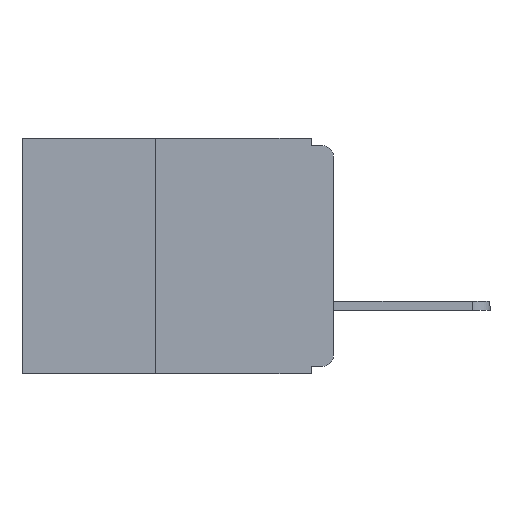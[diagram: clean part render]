
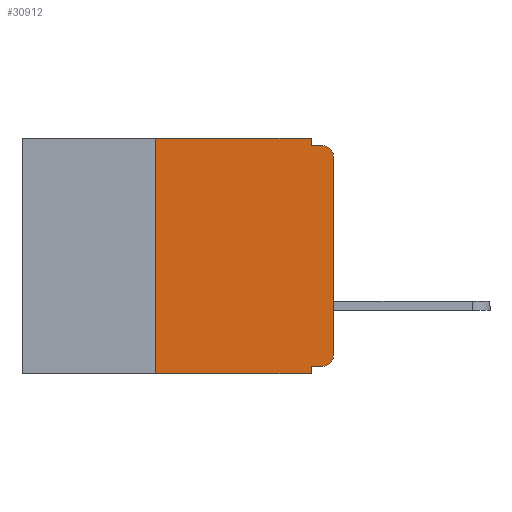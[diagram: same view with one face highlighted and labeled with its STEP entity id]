
A CAD part, left-side view. The second image highlights one B-rep face of the part: STEP entity #30912.
In plain terms, the highlighted planar face has unit normal (-1, 0, 0).
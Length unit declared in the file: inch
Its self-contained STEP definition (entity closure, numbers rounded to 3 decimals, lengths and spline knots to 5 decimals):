
#109 = VECTOR ( 'NONE', #897, 39.37008 ) ;
#129 = EDGE_CURVE ( 'NONE', #1463, #26677, #25511, .T. ) ;
#271 = CIRCLE ( 'NONE', #17665, 0.015 ) ;
#897 = DIRECTION ( 'NONE',  ( 0., -1., 0. ) ) ;
#1276 = CARTESIAN_POINT ( 'NONE',  ( 0., 0.437, 0. ) ) ;
#1463 = VERTEX_POINT ( 'NONE', #8381 ) ;
#1891 = VERTEX_POINT ( 'NONE', #27932 ) ;
#1953 = CARTESIAN_POINT ( 'NONE',  ( 0., 0.25, -0.33 ) ) ;
#1995 = VECTOR ( 'NONE', #17846, 39.37008 ) ;
#2007 = EDGE_CURVE ( 'NONE', #23393, #1891, #16074, .T. ) ;
#2050 = ORIENTED_EDGE ( 'NONE', *, *, #2007, .T. ) ;
#2158 = DIRECTION ( 'NONE',  ( 0., 1., 0. ) ) ;
#3282 = DIRECTION ( 'NONE',  ( -1., 0., 0. ) ) ;
#3568 = CARTESIAN_POINT ( 'NONE',  ( 0., 0., -0.32 ) ) ;
#3985 = PLANE ( 'NONE',  #30162 ) ;
#4313 = ORIENTED_EDGE ( 'NONE', *, *, #6724, .F. ) ;
#4957 = DIRECTION ( 'NONE',  ( -1., 0., 0. ) ) ;
#6204 = CARTESIAN_POINT ( 'NONE',  ( 0., 0., -0.025 ) ) ;
#6392 = CARTESIAN_POINT ( 'NONE',  ( 0., 0.437, 0. ) ) ;
#6442 = CARTESIAN_POINT ( 'NONE',  ( 0., 0.031, -0.01 ) ) ;
#6724 = EDGE_CURVE ( 'NONE', #17417, #29767, #19961, .T. ) ;
#8207 = EDGE_CURVE ( 'NONE', #9996, #31850, #22974, .T. ) ;
#8246 = EDGE_CURVE ( 'NONE', #29767, #15991, #8334, .T. ) ;
#8334 = LINE ( 'NONE', #20729, #16534 ) ;
#8381 = CARTESIAN_POINT ( 'NONE',  ( 0., 0.015, -0.32 ) ) ;
#8713 = ORIENTED_EDGE ( 'NONE', *, *, #18655, .F. ) ;
#9397 = EDGE_CURVE ( 'NONE', #26677, #1891, #15300, .T. ) ;
#9720 = EDGE_CURVE ( 'NONE', #26166, #9996, #25549, .T. ) ;
#9996 = VERTEX_POINT ( 'NONE', #6204 ) ;
#10165 = CARTESIAN_POINT ( 'NONE',  ( 0., 0.015, -0.01 ) ) ;
#10514 = CARTESIAN_POINT ( 'NONE',  ( 0., 0., -0.01 ) ) ;
#10772 = FACE_OUTER_BOUND ( 'NONE', #19765, .T. ) ;
#11352 = LINE ( 'NONE', #10514, #30028 ) ;
#11546 = DIRECTION ( 'NONE',  ( 0., 0., -1. ) ) ;
#11776 = CARTESIAN_POINT ( 'NONE',  ( 0., 0.031, -0.32 ) ) ;
#12889 = ORIENTED_EDGE ( 'NONE', *, *, #129, .F. ) ;
#13146 = AXIS2_PLACEMENT_3D ( 'NONE', #18237, #3282, #20627 ) ;
#15084 = CARTESIAN_POINT ( 'NONE',  ( 0., 0., 0. ) ) ;
#15300 = LINE ( 'NONE', #24915, #1995 ) ;
#15842 = DIRECTION ( 'NONE',  ( 0., 0., -1. ) ) ;
#15991 = VERTEX_POINT ( 'NONE', #6442 ) ;
#16074 = LINE ( 'NONE', #26288, #21785 ) ;
#16534 = VECTOR ( 'NONE', #15842, 39.37008 ) ;
#17417 = VERTEX_POINT ( 'NONE', #31281 ) ;
#17665 = AXIS2_PLACEMENT_3D ( 'NONE', #19818, #4957, #22252 ) ;
#17846 = DIRECTION ( 'NONE',  ( 0., 0., -1. ) ) ;
#18237 = CARTESIAN_POINT ( 'NONE',  ( 0., 0.015, -0.025 ) ) ;
#18655 = EDGE_CURVE ( 'NONE', #23393, #17417, #20930, .T. ) ;
#19062 = VECTOR ( 'NONE', #2158, 39.37008 ) ;
#19101 = VECTOR ( 'NONE', #27195, 39.37008 ) ;
#19765 = EDGE_LOOP ( 'NONE', ( #24061, #22422, #25216, #31058, #4313, #8713, #2050, #29137, #12889, #22709 ) ) ;
#19818 = CARTESIAN_POINT ( 'NONE',  ( 0., 0.015, -0.305 ) ) ;
#19961 = LINE ( 'NONE', #1276, #109 ) ;
#20189 = EDGE_CURVE ( 'NONE', #15991, #31850, #11352, .T. ) ;
#20387 = DIRECTION ( 'NONE',  ( 0., -1., 0. ) ) ;
#20627 = DIRECTION ( 'NONE',  ( 0., 0., -1. ) ) ;
#20729 = CARTESIAN_POINT ( 'NONE',  ( 0., 0.031, 0. ) ) ;
#20930 = LINE ( 'NONE', #1953, #22449 ) ;
#21464 = EDGE_CURVE ( 'NONE', #1463, #26166, #271, .T. ) ;
#21784 = DIRECTION ( 'NONE',  ( 0., 0., 1. ) ) ;
#21785 = VECTOR ( 'NONE', #26042, 39.37008 ) ;
#21978 = CARTESIAN_POINT ( 'NONE',  ( 0., 0., -0.305 ) ) ;
#22252 = DIRECTION ( 'NONE',  ( 0., 0., -1. ) ) ;
#22422 = ORIENTED_EDGE ( 'NONE', *, *, #8207, .T. ) ;
#22449 = VECTOR ( 'NONE', #21784, 39.37008 ) ;
#22709 = ORIENTED_EDGE ( 'NONE', *, *, #21464, .T. ) ;
#22974 = CIRCLE ( 'NONE', #13146, 0.015 ) ;
#23393 = VERTEX_POINT ( 'NONE', #29748 ) ;
#24061 = ORIENTED_EDGE ( 'NONE', *, *, #9720, .T. ) ;
#24915 = CARTESIAN_POINT ( 'NONE',  ( 0., 0.031, -0.33 ) ) ;
#25216 = ORIENTED_EDGE ( 'NONE', *, *, #20189, .F. ) ;
#25511 = LINE ( 'NONE', #3568, #19062 ) ;
#25549 = LINE ( 'NONE', #15084, #19101 ) ;
#26042 = DIRECTION ( 'NONE',  ( 0., -1., 0. ) ) ;
#26166 = VERTEX_POINT ( 'NONE', #21978 ) ;
#26198 = DIRECTION ( 'NONE',  ( 1., 0., 0. ) ) ;
#26288 = CARTESIAN_POINT ( 'NONE',  ( 0., 0.437, -0.33 ) ) ;
#26677 = VERTEX_POINT ( 'NONE', #11776 ) ;
#27195 = DIRECTION ( 'NONE',  ( 0., 0., 1. ) ) ;
#27932 = CARTESIAN_POINT ( 'NONE',  ( 0., 0.031, -0.33 ) ) ;
#28563 = CARTESIAN_POINT ( 'NONE',  ( 0., 0.031, 0. ) ) ;
#29137 = ORIENTED_EDGE ( 'NONE', *, *, #9397, .F. ) ;
#29748 = CARTESIAN_POINT ( 'NONE',  ( 0., 0.25, -0.33 ) ) ;
#29767 = VERTEX_POINT ( 'NONE', #28563 ) ;
#30028 = VECTOR ( 'NONE', #20387, 39.37008 ) ;
#30162 = AXIS2_PLACEMENT_3D ( 'NONE', #6392, #26198, #11546 ) ;
#30912 = ADVANCED_FACE ( 'NONE', ( #10772 ), #3985, .F. ) ;
#31058 = ORIENTED_EDGE ( 'NONE', *, *, #8246, .F. ) ;
#31281 = CARTESIAN_POINT ( 'NONE',  ( 0., 0.25, 0. ) ) ;
#31850 = VERTEX_POINT ( 'NONE', #10165 ) ;
